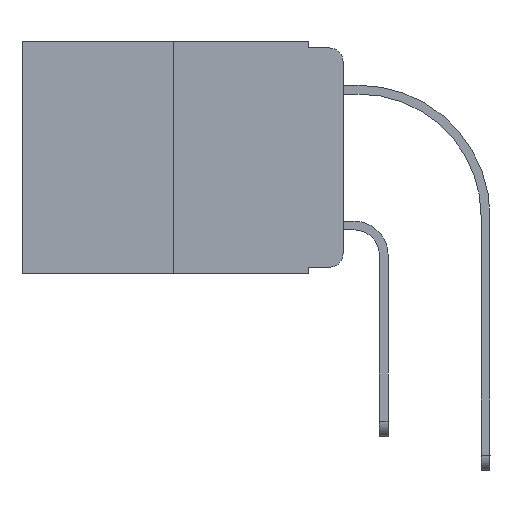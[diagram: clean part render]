
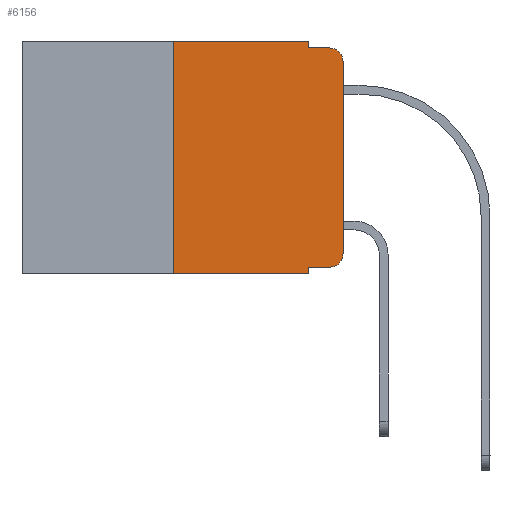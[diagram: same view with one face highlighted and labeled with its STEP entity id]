
A CAD part, left-side view. The second image highlights one B-rep face of the part: STEP entity #6156.
In plain terms, the highlighted planar face has unit normal (-1, 0, 0).
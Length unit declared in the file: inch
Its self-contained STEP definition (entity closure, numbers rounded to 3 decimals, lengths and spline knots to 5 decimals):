
#232 = CARTESIAN_POINT ( 'NONE',  ( 0., 0., -0.313 ) ) ;
#811 = EDGE_CURVE ( 'NONE', #5686, #4188, #17626, .T. ) ;
#857 = DIRECTION ( 'NONE',  ( 0., -1., 0. ) ) ;
#1288 = DIRECTION ( 'NONE',  ( 0., 0., 1. ) ) ;
#1655 = CARTESIAN_POINT ( 'NONE',  ( 0., 0.051, -0.01 ) ) ;
#1944 = CARTESIAN_POINT ( 'NONE',  ( 0., 0.051, -0.333 ) ) ;
#1978 = EDGE_CURVE ( 'NONE', #14055, #17607, #14694, .T. ) ;
#2056 = VECTOR ( 'NONE', #6085, 39.37008 ) ;
#2309 = ORIENTED_EDGE ( 'NONE', *, *, #17538, .T. ) ;
#2379 = CARTESIAN_POINT ( 'NONE',  ( 0., 0.051, -0.333 ) ) ;
#2484 = CARTESIAN_POINT ( 'NONE',  ( 0., 0.02, -0.313 ) ) ;
#2618 = EDGE_CURVE ( 'NONE', #14055, #4188, #12369, .T. ) ;
#3257 = EDGE_CURVE ( 'NONE', #15431, #11429, #10621, .T. ) ;
#3263 = EDGE_CURVE ( 'NONE', #17607, #14832, #7064, .T. ) ;
#3572 = EDGE_CURVE ( 'NONE', #9577, #15263, #16113, .T. ) ;
#3779 = CARTESIAN_POINT ( 'NONE',  ( 0., 0.051, 0. ) ) ;
#4035 = FACE_OUTER_BOUND ( 'NONE', #6007, .T. ) ;
#4185 = DIRECTION ( 'NONE',  ( -1., 0., 0. ) ) ;
#4188 = VERTEX_POINT ( 'NONE', #9082 ) ;
#4314 = DIRECTION ( 'NONE',  ( 0., -1., 0. ) ) ;
#4330 = DIRECTION ( 'NONE',  ( 1., 0., 0. ) ) ;
#4338 = ORIENTED_EDGE ( 'NONE', *, *, #2618, .T. ) ;
#4424 = CARTESIAN_POINT ( 'NONE',  ( 0., 0.051, 0. ) ) ;
#4480 = VECTOR ( 'NONE', #4314, 39.37008 ) ;
#4691 = EDGE_CURVE ( 'NONE', #5686, #15431, #11723, .T. ) ;
#5686 = VERTEX_POINT ( 'NONE', #1944 ) ;
#5746 = CARTESIAN_POINT ( 'NONE',  ( 0., 0.25, 0. ) ) ;
#6007 = EDGE_LOOP ( 'NONE', ( #2309, #10396, #7707, #17748, #17465, #7025, #4338, #8507, #7658, #18267 ) ) ;
#6085 = DIRECTION ( 'NONE',  ( 0., -1., 0. ) ) ;
#6138 = CARTESIAN_POINT ( 'NONE',  ( 0., 0., -0.03 ) ) ;
#6156 = ADVANCED_FACE ( 'NONE', ( #4035 ), #19563, .F. ) ;
#6902 = VECTOR ( 'NONE', #13578, 39.37008 ) ;
#7025 = ORIENTED_EDGE ( 'NONE', *, *, #1978, .F. ) ;
#7064 = LINE ( 'NONE', #14908, #4480 ) ;
#7122 = LINE ( 'NONE', #3779, #18150 ) ;
#7154 = DIRECTION ( 'NONE',  ( -1., 0., 0. ) ) ;
#7586 = CARTESIAN_POINT ( 'NONE',  ( 0., 0.25, 0. ) ) ;
#7658 = ORIENTED_EDGE ( 'NONE', *, *, #4691, .T. ) ;
#7707 = ORIENTED_EDGE ( 'NONE', *, *, #3572, .F. ) ;
#7951 = CARTESIAN_POINT ( 'NONE',  ( 0., 0.051, -0.01 ) ) ;
#8507 = ORIENTED_EDGE ( 'NONE', *, *, #811, .F. ) ;
#9082 = CARTESIAN_POINT ( 'NONE',  ( 0., 0.051, -0.343 ) ) ;
#9138 = CARTESIAN_POINT ( 'NONE',  ( 0., 0.02, -0.01 ) ) ;
#9358 = CARTESIAN_POINT ( 'NONE',  ( 0., 0.25, -0.343 ) ) ;
#9577 = VERTEX_POINT ( 'NONE', #1655 ) ;
#9785 = VERTEX_POINT ( 'NONE', #6138 ) ;
#10390 = DIRECTION ( 'NONE',  ( 0., 0., -1. ) ) ;
#10396 = ORIENTED_EDGE ( 'NONE', *, *, #19137, .T. ) ;
#10548 = EDGE_CURVE ( 'NONE', #14832, #9577, #7122, .T. ) ;
#10596 = AXIS2_PLACEMENT_3D ( 'NONE', #19671, #4330, #16844 ) ;
#10621 = CIRCLE ( 'NONE', #16828, 0.02 ) ;
#11158 = CIRCLE ( 'NONE', #13771, 0.02 ) ;
#11383 = CARTESIAN_POINT ( 'NONE',  ( 0., 0.02, -0.333 ) ) ;
#11429 = VERTEX_POINT ( 'NONE', #232 ) ;
#11527 = DIRECTION ( 'NONE',  ( 0., 0., -1. ) ) ;
#11723 = LINE ( 'NONE', #2379, #12243 ) ;
#12243 = VECTOR ( 'NONE', #857, 39.37008 ) ;
#12369 = LINE ( 'NONE', #13817, #2056 ) ;
#12499 = VECTOR ( 'NONE', #14275, 39.37008 ) ;
#13335 = DIRECTION ( 'NONE',  ( 0., 0., -1. ) ) ;
#13336 = DIRECTION ( 'NONE',  ( 0., 0., -1. ) ) ;
#13578 = DIRECTION ( 'NONE',  ( 0., 0., 1. ) ) ;
#13771 = AXIS2_PLACEMENT_3D ( 'NONE', #15065, #4185, #13335 ) ;
#13817 = CARTESIAN_POINT ( 'NONE',  ( 0., 0.473, -0.343 ) ) ;
#13906 = LINE ( 'NONE', #19980, #14494 ) ;
#14055 = VERTEX_POINT ( 'NONE', #9358 ) ;
#14275 = DIRECTION ( 'NONE',  ( 0., -1., 0. ) ) ;
#14494 = VECTOR ( 'NONE', #1288, 39.37008 ) ;
#14682 = VECTOR ( 'NONE', #11527, 39.37008 ) ;
#14694 = LINE ( 'NONE', #5746, #6902 ) ;
#14809 = CARTESIAN_POINT ( 'NONE',  ( 0., 0.051, 0. ) ) ;
#14832 = VERTEX_POINT ( 'NONE', #4424 ) ;
#14908 = CARTESIAN_POINT ( 'NONE',  ( 0., 0.473, 0. ) ) ;
#15065 = CARTESIAN_POINT ( 'NONE',  ( 0., 0.02, -0.03 ) ) ;
#15263 = VERTEX_POINT ( 'NONE', #9138 ) ;
#15431 = VERTEX_POINT ( 'NONE', #11383 ) ;
#16113 = LINE ( 'NONE', #7951, #12499 ) ;
#16828 = AXIS2_PLACEMENT_3D ( 'NONE', #2484, #7154, #10390 ) ;
#16844 = DIRECTION ( 'NONE',  ( 0., 0., -1. ) ) ;
#17465 = ORIENTED_EDGE ( 'NONE', *, *, #3263, .F. ) ;
#17538 = EDGE_CURVE ( 'NONE', #11429, #9785, #13906, .T. ) ;
#17607 = VERTEX_POINT ( 'NONE', #7586 ) ;
#17626 = LINE ( 'NONE', #14809, #14682 ) ;
#17748 = ORIENTED_EDGE ( 'NONE', *, *, #10548, .F. ) ;
#18150 = VECTOR ( 'NONE', #13336, 39.37008 ) ;
#18267 = ORIENTED_EDGE ( 'NONE', *, *, #3257, .T. ) ;
#19137 = EDGE_CURVE ( 'NONE', #9785, #15263, #11158, .T. ) ;
#19563 = PLANE ( 'NONE',  #10596 ) ;
#19671 = CARTESIAN_POINT ( 'NONE',  ( 0., 0.473, 0. ) ) ;
#19980 = CARTESIAN_POINT ( 'NONE',  ( 0., 0., 0. ) ) ;
